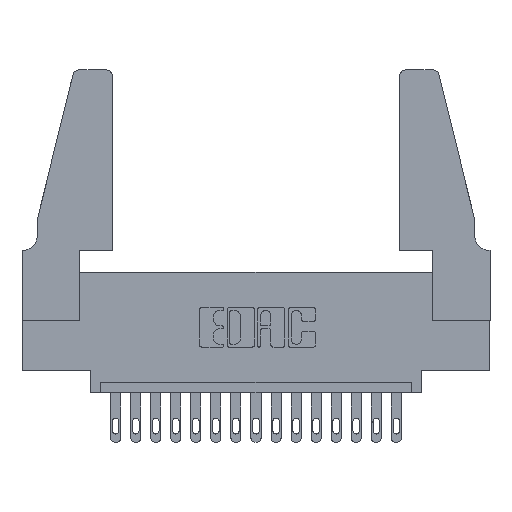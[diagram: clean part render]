
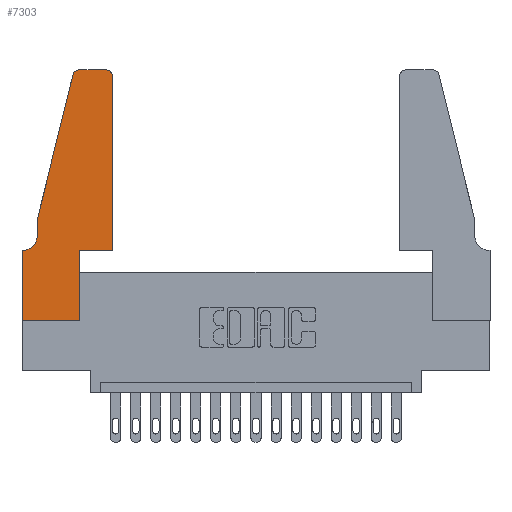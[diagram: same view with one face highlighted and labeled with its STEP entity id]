
A CAD part, top view. The second image highlights one B-rep face of the part: STEP entity #7303.
In plain terms, the highlighted planar face has unit normal (0, 0, 1).
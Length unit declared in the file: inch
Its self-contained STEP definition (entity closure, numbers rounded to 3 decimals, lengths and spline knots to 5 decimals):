
#60 = DIRECTION ( 'NONE',  ( 0., 1., 0. ) ) ;
#228 = CIRCLE ( 'NONE', #14212, 0.07 ) ;
#763 = EDGE_CURVE ( 'NONE', #8318, #1735, #2058, .T. ) ;
#1020 = CARTESIAN_POINT ( 'NONE',  ( 0.25487, 1.22718, 0.37 ) ) ;
#1039 = DIRECTION ( 'NONE',  ( 1., 0., 0. ) ) ;
#1055 = CARTESIAN_POINT ( 'NONE',  ( 0., 0.35, 0.37 ) ) ;
#1238 = LINE ( 'NONE', #6493, #14462 ) ;
#1735 = VERTEX_POINT ( 'NONE', #7231 ) ;
#1809 = VERTEX_POINT ( 'NONE', #16408 ) ;
#1847 = VERTEX_POINT ( 'NONE', #16356 ) ;
#1910 = VERTEX_POINT ( 'NONE', #14116 ) ;
#2058 = LINE ( 'NONE', #16060, #10566 ) ;
#2218 = EDGE_CURVE ( 'NONE', #11684, #13112, #5338, .T. ) ;
#2299 = EDGE_LOOP ( 'NONE', ( #7643, #14125, #10851, #5085, #4022, #10209, #14984, #5795, #9462, #9564, #13484, #14144 ) ) ;
#2362 = CIRCLE ( 'NONE', #13301, 0.03 ) ;
#2427 = LINE ( 'NONE', #14633, #10942 ) ;
#2678 = EDGE_CURVE ( 'NONE', #1847, #1809, #2427, .T. ) ;
#2763 = EDGE_CURVE ( 'NONE', #1910, #8318, #10306, .T. ) ;
#2830 = LINE ( 'NONE', #6486, #16492 ) ;
#2862 = VECTOR ( 'NONE', #3412, 39.37008 ) ;
#3260 = VECTOR ( 'NONE', #4109, 39.37008 ) ;
#3412 = DIRECTION ( 'NONE',  ( 0., 1., 0. ) ) ;
#3496 = VERTEX_POINT ( 'NONE', #1020 ) ;
#3788 = FACE_OUTER_BOUND ( 'NONE', #2299, .T. ) ;
#4022 = ORIENTED_EDGE ( 'NONE', *, *, #6160, .T. ) ;
#4109 = DIRECTION ( 'NONE',  ( 1., 0., 0. ) ) ;
#4251 = DIRECTION ( 'NONE',  ( 0., -1., 0. ) ) ;
#4521 = CARTESIAN_POINT ( 'NONE',  ( 0.0755, 0.5, 0.37 ) ) ;
#4545 = CARTESIAN_POINT ( 'NONE',  ( 0.0055, 0.42, 0.37 ) ) ;
#5059 = VERTEX_POINT ( 'NONE', #12635 ) ;
#5085 = ORIENTED_EDGE ( 'NONE', *, *, #14066, .T. ) ;
#5240 = CARTESIAN_POINT ( 'NONE',  ( 0.4205, 1.22, 0.37 ) ) ;
#5338 = LINE ( 'NONE', #10736, #3260 ) ;
#5618 = CARTESIAN_POINT ( 'NONE',  ( 0.4505, 0.35, 0.37 ) ) ;
#5795 = ORIENTED_EDGE ( 'NONE', *, *, #11530, .T. ) ;
#5949 = CARTESIAN_POINT ( 'NONE',  ( 0., 0.35, 0.37 ) ) ;
#6160 = EDGE_CURVE ( 'NONE', #15758, #1910, #228, .T. ) ;
#6299 = VECTOR ( 'NONE', #60, 39.37008 ) ;
#6414 = CARTESIAN_POINT ( 'NONE',  ( 0.2865, 0.35, 0.37 ) ) ;
#6486 = CARTESIAN_POINT ( 'NONE',  ( 0., 0., 0.37 ) ) ;
#6493 = CARTESIAN_POINT ( 'NONE',  ( 0.0755, 0.5, 0.37 ) ) ;
#6626 = EDGE_CURVE ( 'NONE', #5059, #11684, #13085, .T. ) ;
#6946 = DIRECTION ( 'NONE',  ( 0., -1., 0. ) ) ;
#7231 = CARTESIAN_POINT ( 'NONE',  ( 0., 0., 0.37 ) ) ;
#7303 = ADVANCED_FACE ( 'NONE', ( #3788 ), #12422, .T. ) ;
#7639 = AXIS2_PLACEMENT_3D ( 'NONE', #5240, #13081, #14605 ) ;
#7643 = ORIENTED_EDGE ( 'NONE', *, *, #2678, .T. ) ;
#7761 = VECTOR ( 'NONE', #4251, 39.37008 ) ;
#8090 = DIRECTION ( 'NONE',  ( 1., 0., 0. ) ) ;
#8318 = VERTEX_POINT ( 'NONE', #1055 ) ;
#8791 = EDGE_CURVE ( 'NONE', #16942, #1847, #9998, .T. ) ;
#9174 = CARTESIAN_POINT ( 'NONE',  ( 0.0755, 0.5, 0.37 ) ) ;
#9462 = ORIENTED_EDGE ( 'NONE', *, *, #6626, .T. ) ;
#9564 = ORIENTED_EDGE ( 'NONE', *, *, #2218, .T. ) ;
#9851 = EDGE_CURVE ( 'NONE', #3496, #14244, #1238, .T. ) ;
#9998 = CIRCLE ( 'NONE', #7639, 0.03 ) ;
#10209 = ORIENTED_EDGE ( 'NONE', *, *, #2763, .T. ) ;
#10263 = EDGE_CURVE ( 'NONE', #13112, #16942, #13394, .T. ) ;
#10306 = LINE ( 'NONE', #16281, #10925 ) ;
#10320 = DIRECTION ( 'NONE',  ( -0.239, -0.971, 0. ) ) ;
#10442 = LINE ( 'NONE', #9174, #7761 ) ;
#10566 = VECTOR ( 'NONE', #6946, 39.37008 ) ;
#10736 = CARTESIAN_POINT ( 'NONE',  ( 0.4505, 0.35, 0.37 ) ) ;
#10851 = ORIENTED_EDGE ( 'NONE', *, *, #9851, .T. ) ;
#10925 = VECTOR ( 'NONE', #13433, 39.37008 ) ;
#10942 = VECTOR ( 'NONE', #13342, 39.37008 ) ;
#11530 = EDGE_CURVE ( 'NONE', #1735, #5059, #2830, .T. ) ;
#11684 = VERTEX_POINT ( 'NONE', #13090 ) ;
#12422 = PLANE ( 'NONE',  #13784 ) ;
#12635 = CARTESIAN_POINT ( 'NONE',  ( 0.2865, 0., 0.37 ) ) ;
#12982 = CARTESIAN_POINT ( 'NONE',  ( 0.0755, 0.42, 0.37 ) ) ;
#13081 = DIRECTION ( 'NONE',  ( 0., 0., 1. ) ) ;
#13085 = LINE ( 'NONE', #6414, #6299 ) ;
#13090 = CARTESIAN_POINT ( 'NONE',  ( 0.2865, 0.35, 0.37 ) ) ;
#13112 = VERTEX_POINT ( 'NONE', #5618 ) ;
#13301 = AXIS2_PLACEMENT_3D ( 'NONE', #14549, #14491, #8090 ) ;
#13342 = DIRECTION ( 'NONE',  ( -1., 0., 0. ) ) ;
#13394 = LINE ( 'NONE', #16725, #2862 ) ;
#13433 = DIRECTION ( 'NONE',  ( -1., 0., 0. ) ) ;
#13484 = ORIENTED_EDGE ( 'NONE', *, *, #10263, .T. ) ;
#13512 = EDGE_CURVE ( 'NONE', #1809, #3496, #2362, .T. ) ;
#13784 = AXIS2_PLACEMENT_3D ( 'NONE', #5949, #15185, #16578 ) ;
#14066 = EDGE_CURVE ( 'NONE', #14244, #15758, #10442, .T. ) ;
#14116 = CARTESIAN_POINT ( 'NONE',  ( 0.0055, 0.35, 0.37 ) ) ;
#14125 = ORIENTED_EDGE ( 'NONE', *, *, #13512, .T. ) ;
#14144 = ORIENTED_EDGE ( 'NONE', *, *, #8791, .T. ) ;
#14212 = AXIS2_PLACEMENT_3D ( 'NONE', #4545, #14438, #17079 ) ;
#14244 = VERTEX_POINT ( 'NONE', #4521 ) ;
#14438 = DIRECTION ( 'NONE',  ( 0., 0., -1. ) ) ;
#14462 = VECTOR ( 'NONE', #10320, 39.37008 ) ;
#14491 = DIRECTION ( 'NONE',  ( 0., 0., 1. ) ) ;
#14549 = CARTESIAN_POINT ( 'NONE',  ( 0.284, 1.22, 0.37 ) ) ;
#14573 = CARTESIAN_POINT ( 'NONE',  ( 0.4505, 1.22, 0.37 ) ) ;
#14605 = DIRECTION ( 'NONE',  ( 1., 0., 0. ) ) ;
#14633 = CARTESIAN_POINT ( 'NONE',  ( 0.2605, 1.25, 0.37 ) ) ;
#14984 = ORIENTED_EDGE ( 'NONE', *, *, #763, .T. ) ;
#15185 = DIRECTION ( 'NONE',  ( 0., 0., 1. ) ) ;
#15758 = VERTEX_POINT ( 'NONE', #12982 ) ;
#16060 = CARTESIAN_POINT ( 'NONE',  ( 0., 0., 0.37 ) ) ;
#16281 = CARTESIAN_POINT ( 'NONE',  ( 0.0755, 0.35, 0.37 ) ) ;
#16356 = CARTESIAN_POINT ( 'NONE',  ( 0.4205, 1.25, 0.37 ) ) ;
#16408 = CARTESIAN_POINT ( 'NONE',  ( 0.284, 1.25, 0.37 ) ) ;
#16492 = VECTOR ( 'NONE', #1039, 39.37008 ) ;
#16578 = DIRECTION ( 'NONE',  ( 1., 0., 0. ) ) ;
#16725 = CARTESIAN_POINT ( 'NONE',  ( 0.4505, 0.35, 0.37 ) ) ;
#16942 = VERTEX_POINT ( 'NONE', #14573 ) ;
#17079 = DIRECTION ( 'NONE',  ( -1., 0., 0. ) ) ;
